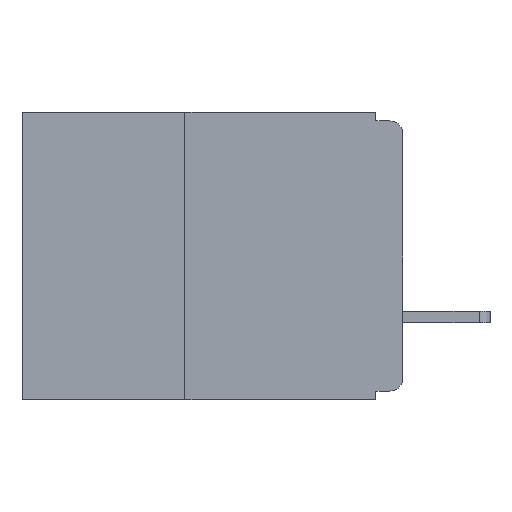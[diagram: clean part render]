
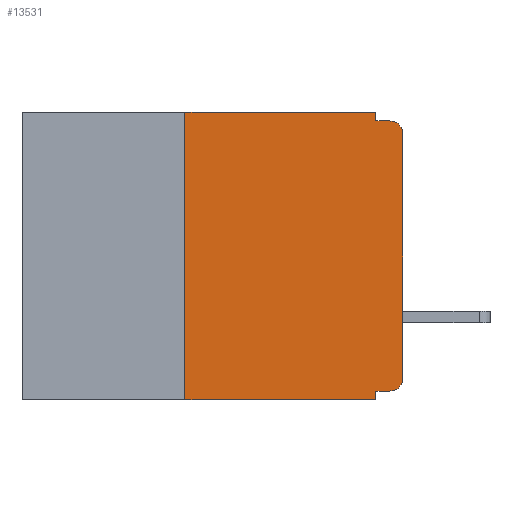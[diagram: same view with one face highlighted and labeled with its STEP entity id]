
A CAD part, left-side view. The second image highlights one B-rep face of the part: STEP entity #13531.
In plain terms, the highlighted planar face has unit normal (-1, 0, 0).
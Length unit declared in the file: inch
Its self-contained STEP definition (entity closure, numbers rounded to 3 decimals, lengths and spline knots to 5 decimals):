
#307 = DIRECTION ( 'NONE',  ( 0., 0., -1. ) ) ;
#348 = VERTEX_POINT ( 'NONE', #5951 ) ;
#1053 = DIRECTION ( 'NONE',  ( 1., 0., 0. ) ) ;
#1175 = CARTESIAN_POINT ( 'NONE',  ( 0., 0.031, 0. ) ) ;
#1689 = VERTEX_POINT ( 'NONE', #12262 ) ;
#1744 = VECTOR ( 'NONE', #12928, 39.37008 ) ;
#1838 = LINE ( 'NONE', #12637, #1744 ) ;
#2093 = DIRECTION ( 'NONE',  ( 0., 0., -1. ) ) ;
#2193 = VECTOR ( 'NONE', #13187, 39.37008 ) ;
#2325 = AXIS2_PLACEMENT_3D ( 'NONE', #8617, #8595, #8556 ) ;
#2481 = LINE ( 'NONE', #13401, #2193 ) ;
#2670 = VECTOR ( 'NONE', #16875, 39.37008 ) ;
#2697 = DIRECTION ( 'NONE',  ( -1., 0., 0. ) ) ;
#2700 = EDGE_CURVE ( 'NONE', #1689, #6622, #7010, .T. ) ;
#2815 = CARTESIAN_POINT ( 'NONE',  ( 0., 0.437, 0. ) ) ;
#2890 = PLANE ( 'NONE',  #6213 ) ;
#2910 = LINE ( 'NONE', #17319, #2670 ) ;
#3430 = CARTESIAN_POINT ( 'NONE',  ( 0., 0.031, 0. ) ) ;
#4269 = DIRECTION ( 'NONE',  ( 0., 0., -1. ) ) ;
#4389 = EDGE_CURVE ( 'NONE', #16413, #1689, #15582, .T. ) ;
#4646 = CARTESIAN_POINT ( 'NONE',  ( 0., 0.031, -0.33 ) ) ;
#4976 = ORIENTED_EDGE ( 'NONE', *, *, #4389, .F. ) ;
#5286 = ORIENTED_EDGE ( 'NONE', *, *, #8410, .T. ) ;
#5651 = ORIENTED_EDGE ( 'NONE', *, *, #6917, .T. ) ;
#5901 = DIRECTION ( 'NONE',  ( 0., -1., 0. ) ) ;
#5951 = CARTESIAN_POINT ( 'NONE',  ( 0., 0., -0.305 ) ) ;
#6004 = VERTEX_POINT ( 'NONE', #12282 ) ;
#6161 = CARTESIAN_POINT ( 'NONE',  ( 0., 0.437, 0. ) ) ;
#6213 = AXIS2_PLACEMENT_3D ( 'NONE', #2815, #1053, #307 ) ;
#6244 = VERTEX_POINT ( 'NONE', #4646 ) ;
#6278 = EDGE_CURVE ( 'NONE', #6622, #11971, #11234, .T. ) ;
#6516 = ORIENTED_EDGE ( 'NONE', *, *, #17106, .F. ) ;
#6622 = VERTEX_POINT ( 'NONE', #1175 ) ;
#6917 = EDGE_CURVE ( 'NONE', #16413, #6244, #8207, .T. ) ;
#6988 = VECTOR ( 'NONE', #5901, 39.37008 ) ;
#7010 = LINE ( 'NONE', #6161, #6988 ) ;
#7129 = CARTESIAN_POINT ( 'NONE',  ( 0., 0., -0.025 ) ) ;
#7690 = EDGE_LOOP ( 'NONE', ( #5286, #14712, #15187, #16554, #15968, #4976, #5651, #6516, #12670, #11816 ) ) ;
#8180 = VECTOR ( 'NONE', #12591, 39.37008 ) ;
#8207 = LINE ( 'NONE', #12512, #8180 ) ;
#8263 = CARTESIAN_POINT ( 'NONE',  ( 0., 0.015, -0.32 ) ) ;
#8313 = VERTEX_POINT ( 'NONE', #16077 ) ;
#8410 = EDGE_CURVE ( 'NONE', #348, #9006, #1838, .T. ) ;
#8556 = DIRECTION ( 'NONE',  ( 0., 0., -1. ) ) ;
#8595 = DIRECTION ( 'NONE',  ( -1., 0., 0. ) ) ;
#8617 = CARTESIAN_POINT ( 'NONE',  ( 0., 0.015, -0.305 ) ) ;
#8951 = VERTEX_POINT ( 'NONE', #8263 ) ;
#9006 = VERTEX_POINT ( 'NONE', #7129 ) ;
#9163 = DIRECTION ( 'NONE',  ( 0., 0., -1. ) ) ;
#9222 = CARTESIAN_POINT ( 'NONE',  ( 0., 0.031, -0.33 ) ) ;
#9394 = CARTESIAN_POINT ( 'NONE',  ( 0., 0.25, -0.33 ) ) ;
#9439 = CARTESIAN_POINT ( 'NONE',  ( 0., 0.015, -0.025 ) ) ;
#10316 = EDGE_CURVE ( 'NONE', #11971, #6004, #2481, .T. ) ;
#11033 = VECTOR ( 'NONE', #4269, 39.37008 ) ;
#11234 = LINE ( 'NONE', #3430, #11033 ) ;
#11816 = ORIENTED_EDGE ( 'NONE', *, *, #17123, .T. ) ;
#11971 = VERTEX_POINT ( 'NONE', #17674 ) ;
#12262 = CARTESIAN_POINT ( 'NONE',  ( 0., 0.25, 0. ) ) ;
#12282 = CARTESIAN_POINT ( 'NONE',  ( 0., 0.015, -0.01 ) ) ;
#12301 = DIRECTION ( 'NONE',  ( 0., 0., 1. ) ) ;
#12351 = CARTESIAN_POINT ( 'NONE',  ( 0., 0.25, -0.33 ) ) ;
#12512 = CARTESIAN_POINT ( 'NONE',  ( 0., 0.437, -0.33 ) ) ;
#12591 = DIRECTION ( 'NONE',  ( 0., -1., 0. ) ) ;
#12637 = CARTESIAN_POINT ( 'NONE',  ( 0., 0., 0. ) ) ;
#12670 = ORIENTED_EDGE ( 'NONE', *, *, #16236, .F. ) ;
#12928 = DIRECTION ( 'NONE',  ( 0., 0., 1. ) ) ;
#13051 = VECTOR ( 'NONE', #9163, 39.37008 ) ;
#13091 = CIRCLE ( 'NONE', #2325, 0.015 ) ;
#13129 = LINE ( 'NONE', #9222, #13051 ) ;
#13187 = DIRECTION ( 'NONE',  ( 0., -1., 0. ) ) ;
#13401 = CARTESIAN_POINT ( 'NONE',  ( 0., 0., -0.01 ) ) ;
#13531 = ADVANCED_FACE ( 'NONE', ( #13628 ), #2890, .F. ) ;
#13628 = FACE_OUTER_BOUND ( 'NONE', #7690, .T. ) ;
#14378 = CIRCLE ( 'NONE', #14779, 0.015 ) ;
#14712 = ORIENTED_EDGE ( 'NONE', *, *, #16906, .T. ) ;
#14779 = AXIS2_PLACEMENT_3D ( 'NONE', #9439, #2697, #2093 ) ;
#15187 = ORIENTED_EDGE ( 'NONE', *, *, #10316, .F. ) ;
#15567 = VECTOR ( 'NONE', #12301, 39.37008 ) ;
#15582 = LINE ( 'NONE', #12351, #15567 ) ;
#15968 = ORIENTED_EDGE ( 'NONE', *, *, #2700, .F. ) ;
#16077 = CARTESIAN_POINT ( 'NONE',  ( 0., 0.031, -0.32 ) ) ;
#16236 = EDGE_CURVE ( 'NONE', #8951, #8313, #2910, .T. ) ;
#16413 = VERTEX_POINT ( 'NONE', #9394 ) ;
#16554 = ORIENTED_EDGE ( 'NONE', *, *, #6278, .F. ) ;
#16875 = DIRECTION ( 'NONE',  ( 0., 1., 0. ) ) ;
#16906 = EDGE_CURVE ( 'NONE', #9006, #6004, #14378, .T. ) ;
#17106 = EDGE_CURVE ( 'NONE', #8313, #6244, #13129, .T. ) ;
#17123 = EDGE_CURVE ( 'NONE', #8951, #348, #13091, .T. ) ;
#17319 = CARTESIAN_POINT ( 'NONE',  ( 0., 0., -0.32 ) ) ;
#17674 = CARTESIAN_POINT ( 'NONE',  ( 0., 0.031, -0.01 ) ) ;
